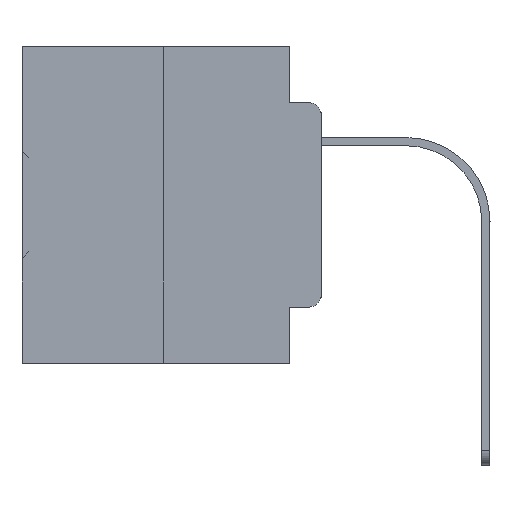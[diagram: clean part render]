
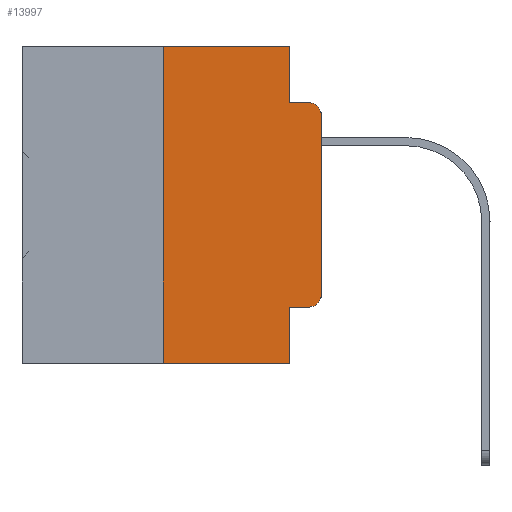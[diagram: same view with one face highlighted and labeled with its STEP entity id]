
A CAD part, left-side view. The second image highlights one B-rep face of the part: STEP entity #13997.
In plain terms, the highlighted planar face has unit normal (-1, 0, 0).
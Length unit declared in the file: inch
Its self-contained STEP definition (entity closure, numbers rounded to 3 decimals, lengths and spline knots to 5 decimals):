
#328 = LINE ( 'NONE', #34257, #9654 ) ;
#478 = VERTEX_POINT ( 'NONE', #8382 ) ;
#1172 = VERTEX_POINT ( 'NONE', #1612 ) ;
#1175 = AXIS2_PLACEMENT_3D ( 'NONE', #15551, #32511, #6959 ) ;
#1189 = LINE ( 'NONE', #21504, #2898 ) ;
#1542 = VERTEX_POINT ( 'NONE', #36561 ) ;
#1612 = CARTESIAN_POINT ( 'NONE',  ( 0., 0.051, -0.0885 ) ) ;
#2257 = EDGE_CURVE ( 'NONE', #19014, #11011, #21529, .T. ) ;
#2760 = ORIENTED_EDGE ( 'NONE', *, *, #3020, .T. ) ;
#2849 = CARTESIAN_POINT ( 'NONE',  ( 0., 0.051, 0. ) ) ;
#2898 = VECTOR ( 'NONE', #32893, 39.37008 ) ;
#3020 = EDGE_CURVE ( 'NONE', #478, #28317, #328, .T. ) ;
#4546 = VECTOR ( 'NONE', #29514, 39.37008 ) ;
#4679 = LINE ( 'NONE', #30397, #19803 ) ;
#5249 = CARTESIAN_POINT ( 'NONE',  ( 0., 0.25, 0. ) ) ;
#5508 = DIRECTION ( 'NONE',  ( 0., 0., -1. ) ) ;
#5546 = CARTESIAN_POINT ( 'NONE',  ( 0., 0.051, -0.0885 ) ) ;
#5966 = VECTOR ( 'NONE', #33115, 39.37008 ) ;
#6410 = AXIS2_PLACEMENT_3D ( 'NONE', #10777, #34065, #19688 ) ;
#6419 = EDGE_CURVE ( 'NONE', #28317, #21795, #30337, .T. ) ;
#6959 = DIRECTION ( 'NONE',  ( 0., 0., -1. ) ) ;
#8382 = CARTESIAN_POINT ( 'NONE',  ( 0., 0.051, -0.4115 ) ) ;
#8889 = DIRECTION ( 'NONE',  ( 0., -1., 0. ) ) ;
#9654 = VECTOR ( 'NONE', #8889, 39.37008 ) ;
#9778 = EDGE_LOOP ( 'NONE', ( #12306, #20067, #11927, #13772, #23571, #26631, #20725, #22165, #2760, #28325 ) ) ;
#10777 = CARTESIAN_POINT ( 'NONE',  ( 0., 0.473, 0. ) ) ;
#11011 = VERTEX_POINT ( 'NONE', #22149 ) ;
#11086 = VECTOR ( 'NONE', #35554, 39.37008 ) ;
#11803 = VECTOR ( 'NONE', #5508, 39.37008 ) ;
#11927 = ORIENTED_EDGE ( 'NONE', *, *, #28978, .F. ) ;
#11947 = VERTEX_POINT ( 'NONE', #5249 ) ;
#12306 = ORIENTED_EDGE ( 'NONE', *, *, #23463, .T. ) ;
#12764 = LINE ( 'NONE', #35517, #4546 ) ;
#12947 = CARTESIAN_POINT ( 'NONE',  ( 0., 0.051, -0.5 ) ) ;
#13772 = ORIENTED_EDGE ( 'NONE', *, *, #14466, .F. ) ;
#13997 = ADVANCED_FACE ( 'NONE', ( #19329 ), #19150, .F. ) ;
#14377 = VERTEX_POINT ( 'NONE', #12947 ) ;
#14466 = EDGE_CURVE ( 'NONE', #27234, #1172, #1189, .T. ) ;
#15075 = CARTESIAN_POINT ( 'NONE',  ( 0., 0., 0. ) ) ;
#15395 = EDGE_CURVE ( 'NONE', #478, #14377, #31049, .T. ) ;
#15551 = CARTESIAN_POINT ( 'NONE',  ( 0., 0.02, -0.3915 ) ) ;
#16752 = LINE ( 'NONE', #5546, #25842 ) ;
#17323 = CARTESIAN_POINT ( 'NONE',  ( 0., 0., -0.1085 ) ) ;
#17883 = CARTESIAN_POINT ( 'NONE',  ( 0., 0., -0.3915 ) ) ;
#18190 = CARTESIAN_POINT ( 'NONE',  ( 0., 0.02, -0.4115 ) ) ;
#19014 = VERTEX_POINT ( 'NONE', #17323 ) ;
#19150 = PLANE ( 'NONE',  #6410 ) ;
#19329 = FACE_OUTER_BOUND ( 'NONE', #9778, .T. ) ;
#19481 = CARTESIAN_POINT ( 'NONE',  ( 0., 0.02, -0.1085 ) ) ;
#19688 = DIRECTION ( 'NONE',  ( 0., 0., -1. ) ) ;
#19803 = VECTOR ( 'NONE', #24235, 39.37008 ) ;
#20067 = ORIENTED_EDGE ( 'NONE', *, *, #2257, .T. ) ;
#20725 = ORIENTED_EDGE ( 'NONE', *, *, #35367, .T. ) ;
#21504 = CARTESIAN_POINT ( 'NONE',  ( 0., 0.051, 0. ) ) ;
#21529 = CIRCLE ( 'NONE', #26863, 0.02 ) ;
#21795 = VERTEX_POINT ( 'NONE', #17883 ) ;
#22149 = CARTESIAN_POINT ( 'NONE',  ( 0., 0.02, -0.0885 ) ) ;
#22165 = ORIENTED_EDGE ( 'NONE', *, *, #15395, .F. ) ;
#23463 = EDGE_CURVE ( 'NONE', #21795, #19014, #35743, .T. ) ;
#23571 = ORIENTED_EDGE ( 'NONE', *, *, #30994, .F. ) ;
#24235 = DIRECTION ( 'NONE',  ( 0., -1., 0. ) ) ;
#25842 = VECTOR ( 'NONE', #28097, 39.37008 ) ;
#26631 = ORIENTED_EDGE ( 'NONE', *, *, #35843, .F. ) ;
#26863 = AXIS2_PLACEMENT_3D ( 'NONE', #19481, #28420, #34769 ) ;
#27234 = VERTEX_POINT ( 'NONE', #2849 ) ;
#28097 = DIRECTION ( 'NONE',  ( 0., -1., 0. ) ) ;
#28317 = VERTEX_POINT ( 'NONE', #18190 ) ;
#28325 = ORIENTED_EDGE ( 'NONE', *, *, #6419, .T. ) ;
#28420 = DIRECTION ( 'NONE',  ( -1., 0., 0. ) ) ;
#28978 = EDGE_CURVE ( 'NONE', #1172, #11011, #16752, .T. ) ;
#29514 = DIRECTION ( 'NONE',  ( 0., 0., 1. ) ) ;
#29940 = LINE ( 'NONE', #35742, #11086 ) ;
#30337 = CIRCLE ( 'NONE', #1175, 0.02 ) ;
#30397 = CARTESIAN_POINT ( 'NONE',  ( 0., 0.473, 0. ) ) ;
#30994 = EDGE_CURVE ( 'NONE', #11947, #27234, #4679, .T. ) ;
#31049 = LINE ( 'NONE', #33488, #11803 ) ;
#32511 = DIRECTION ( 'NONE',  ( -1., 0., 0. ) ) ;
#32893 = DIRECTION ( 'NONE',  ( 0., 0., -1. ) ) ;
#33115 = DIRECTION ( 'NONE',  ( 0., 0., 1. ) ) ;
#33488 = CARTESIAN_POINT ( 'NONE',  ( 0., 0.051, 0. ) ) ;
#34065 = DIRECTION ( 'NONE',  ( 1., 0., 0. ) ) ;
#34257 = CARTESIAN_POINT ( 'NONE',  ( 0., 0.051, -0.4115 ) ) ;
#34769 = DIRECTION ( 'NONE',  ( 0., 0., -1. ) ) ;
#35367 = EDGE_CURVE ( 'NONE', #1542, #14377, #29940, .T. ) ;
#35517 = CARTESIAN_POINT ( 'NONE',  ( 0., 0.25, 0. ) ) ;
#35554 = DIRECTION ( 'NONE',  ( 0., -1., 0. ) ) ;
#35742 = CARTESIAN_POINT ( 'NONE',  ( 0., 0.473, -0.5 ) ) ;
#35743 = LINE ( 'NONE', #15075, #5966 ) ;
#35843 = EDGE_CURVE ( 'NONE', #1542, #11947, #12764, .T. ) ;
#36561 = CARTESIAN_POINT ( 'NONE',  ( 0., 0.25, -0.5 ) ) ;
